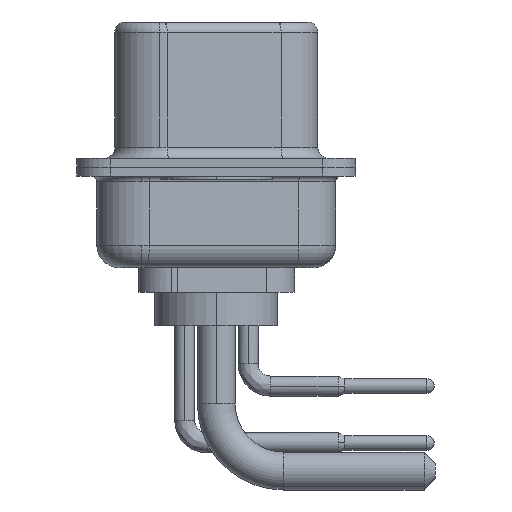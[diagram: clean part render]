
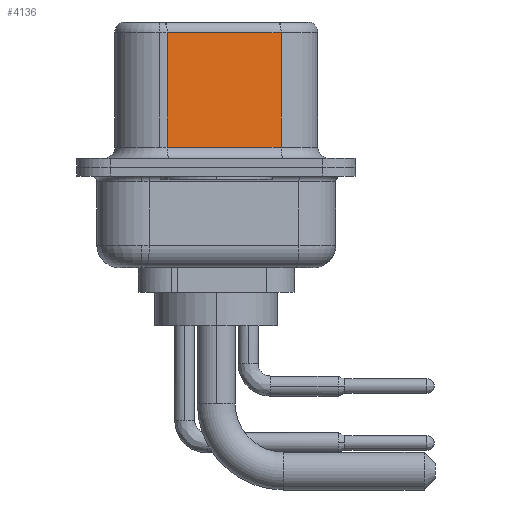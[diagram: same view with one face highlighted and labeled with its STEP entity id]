
A CAD part, left-side view. The second image highlights one B-rep face of the part: STEP entity #4136.
In plain terms, the highlighted planar face has unit normal (-0.985, -0.174, 0).
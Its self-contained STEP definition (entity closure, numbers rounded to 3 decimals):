
#7 = ORIENTED_EDGE ( 'NONE', *, *, #19188, .F. ) ;
#534 = LINE ( 'NONE', #2786, #13406 ) ;
#850 = EDGE_LOOP ( 'NONE', ( #7, #25639, #19086, #7913 ) ) ;
#920 = CARTESIAN_POINT ( 'NONE',  ( 4.58, -2.897, 6.52 ) ) ;
#2307 = VERTEX_POINT ( 'NONE', #25867 ) ;
#2786 = CARTESIAN_POINT ( 'NONE',  ( 4.58, -2.897, 0.9 ) ) ;
#3130 = DIRECTION ( 'NONE',  ( 0., 0., -1. ) ) ;
#4136 = ADVANCED_FACE ( 'NONE', ( #17445 ), #8877, .F. ) ;
#4624 = VERTEX_POINT ( 'NONE', #14912 ) ;
#5122 = CARTESIAN_POINT ( 'NONE',  ( 4.58, -2.897, 6.52 ) ) ;
#7913 = ORIENTED_EDGE ( 'NONE', *, *, #19830, .T. ) ;
#8877 = PLANE ( 'NONE',  #15065 ) ;
#8894 = DIRECTION ( 'NONE',  ( 0.174, -0.985, 0. ) ) ;
#9265 = DIRECTION ( 'NONE',  ( -0.174, 0.985, 0. ) ) ;
#10697 = DIRECTION ( 'NONE',  ( -0.174, 0.985, 0. ) ) ;
#11385 = DIRECTION ( 'NONE',  ( 0., 0., -1. ) ) ;
#12008 = EDGE_CURVE ( 'NONE', #2307, #4624, #14952, .T. ) ;
#13406 = VECTOR ( 'NONE', #8894, 1000. ) ;
#13517 = EDGE_CURVE ( 'NONE', #19788, #2307, #24298, .T. ) ;
#14748 = CARTESIAN_POINT ( 'NONE',  ( 4.58, -2.897, 0.9 ) ) ;
#14912 = CARTESIAN_POINT ( 'NONE',  ( 3.68, 2.203, 0.9 ) ) ;
#14952 = LINE ( 'NONE', #21285, #18467 ) ;
#15065 = AXIS2_PLACEMENT_3D ( 'NONE', #920, #15452, #9265 ) ;
#15185 = LINE ( 'NONE', #5122, #16309 ) ;
#15452 = DIRECTION ( 'NONE',  ( 0.985, 0.174, 0. ) ) ;
#16007 = VECTOR ( 'NONE', #10697, 1000. ) ;
#16309 = VECTOR ( 'NONE', #3130, 1000. ) ;
#17445 = FACE_OUTER_BOUND ( 'NONE', #850, .T. ) ;
#18399 = CARTESIAN_POINT ( 'NONE',  ( 4.58, -2.897, 6.02 ) ) ;
#18467 = VECTOR ( 'NONE', #11385, 1000. ) ;
#19086 = ORIENTED_EDGE ( 'NONE', *, *, #12008, .T. ) ;
#19188 = EDGE_CURVE ( 'NONE', #19788, #24163, #15185, .T. ) ;
#19788 = VERTEX_POINT ( 'NONE', #18399 ) ;
#19830 = EDGE_CURVE ( 'NONE', #4624, #24163, #534, .T. ) ;
#21285 = CARTESIAN_POINT ( 'NONE',  ( 3.68, 2.203, 6.52 ) ) ;
#22179 = CARTESIAN_POINT ( 'NONE',  ( 4.58, -2.897, 6.02 ) ) ;
#24163 = VERTEX_POINT ( 'NONE', #14748 ) ;
#24298 = LINE ( 'NONE', #22179, #16007 ) ;
#25639 = ORIENTED_EDGE ( 'NONE', *, *, #13517, .T. ) ;
#25867 = CARTESIAN_POINT ( 'NONE',  ( 3.68, 2.203, 6.02 ) ) ;
